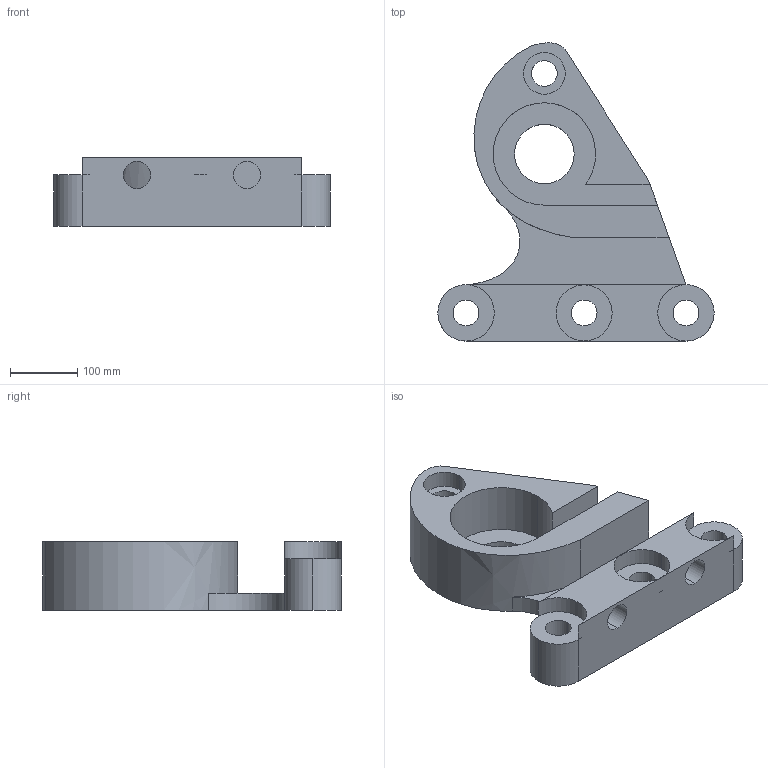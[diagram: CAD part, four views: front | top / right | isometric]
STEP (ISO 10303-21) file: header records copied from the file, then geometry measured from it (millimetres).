
FILE_DESCRIPTION (( 'STEP AP214' ), '1' );
FILE_NAME ('Plate_2.STEP', '2014-02-05T15:25:23', ( 'elpi' ), ( '' ), 'SwSTEP 2.0', 'SolidWorks 2013', '' );
FILE_SCHEMA (( 'AUTOMOTIVE_DESIGN' ));
Length unit declared in the file: inch
Products named in the file (1): Plate_2
Bounding box: 411.04 x 443.66 x 101.6 mm (x, y, z)
Volume: 6455340.1 mm3; surface area: 488500.7 mm2
Topology: 1 solids, 1 shells, 46 faces, 120 edges, 78 vertices
Faces by surface type: cylinder 27, plane 16, bspline 3
Entity records: 1513 total; most frequent: CARTESIAN_POINT 283, DIRECTION 255, ORIENTED_EDGE 240, EDGE_CURVE 120, AXIS2_PLACEMENT_3D 98, VERTEX_POINT 78, EDGE_LOOP 62, LINE 59
